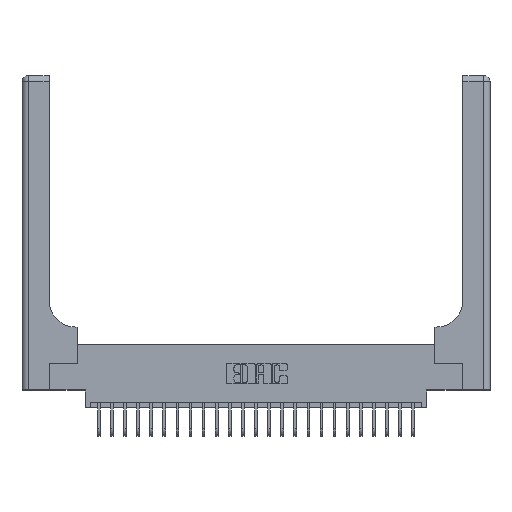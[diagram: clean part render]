
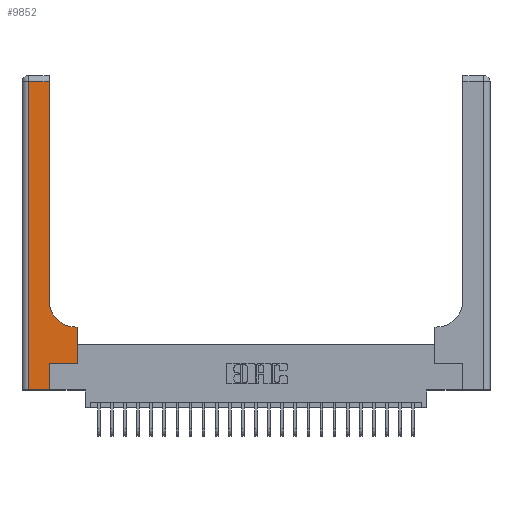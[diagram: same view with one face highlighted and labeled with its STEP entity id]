
A CAD part, top view. The second image highlights one B-rep face of the part: STEP entity #9852.
In plain terms, the highlighted planar face has unit normal (0, 0, 1).
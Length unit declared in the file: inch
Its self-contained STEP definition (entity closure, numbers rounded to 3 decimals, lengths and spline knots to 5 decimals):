
#57 = CARTESIAN_POINT ( 'NONE',  ( 0.06, 0., 0.37 ) ) ;
#827 = CARTESIAN_POINT ( 'NONE',  ( 0.26, 0.6, 0.37 ) ) ;
#976 = CARTESIAN_POINT ( 'NONE',  ( 0., 2.94, 0.37 ) ) ;
#1047 = DIRECTION ( 'NONE',  ( 0., 1., 0. ) ) ;
#1135 = DIRECTION ( 'NONE',  ( 0., 1., 0. ) ) ;
#1375 = LINE ( 'NONE', #8776, #22037 ) ;
#1558 = DIRECTION ( 'NONE',  ( 1., 0., 0. ) ) ;
#1727 = VERTEX_POINT ( 'NONE', #16387 ) ;
#2188 = VERTEX_POINT ( 'NONE', #4169 ) ;
#2196 = DIRECTION ( 'NONE',  ( 0., 1., 0. ) ) ;
#2370 = ORIENTED_EDGE ( 'NONE', *, *, #7358, .T. ) ;
#2479 = VERTEX_POINT ( 'NONE', #57 ) ;
#2896 = VECTOR ( 'NONE', #8259, 39.37008 ) ;
#3186 = ORIENTED_EDGE ( 'NONE', *, *, #9248, .T. ) ;
#3630 = ORIENTED_EDGE ( 'NONE', *, *, #19586, .T. ) ;
#3804 = CARTESIAN_POINT ( 'NONE',  ( 0.265, 0.25, 0.37 ) ) ;
#3867 = PLANE ( 'NONE',  #10212 ) ;
#4169 = CARTESIAN_POINT ( 'NONE',  ( 0.06, 2.94, 0.37 ) ) ;
#4468 = LINE ( 'NONE', #18923, #5776 ) ;
#4624 = VECTOR ( 'NONE', #9893, 39.37008 ) ;
#5185 = AXIS2_PLACEMENT_3D ( 'NONE', #12071, #22974, #1558 ) ;
#5554 = DIRECTION ( 'NONE',  ( -1., 0., 0. ) ) ;
#5571 = CARTESIAN_POINT ( 'NONE',  ( 0.265, 0., 0.37 ) ) ;
#5776 = VECTOR ( 'NONE', #2196, 39.37008 ) ;
#6435 = VERTEX_POINT ( 'NONE', #3804 ) ;
#6453 = CARTESIAN_POINT ( 'NONE',  ( 0.528, 0.25, 0.37 ) ) ;
#7325 = EDGE_CURVE ( 'NONE', #1727, #2188, #17358, .T. ) ;
#7358 = EDGE_CURVE ( 'NONE', #7975, #13155, #16233, .T. ) ;
#7469 = VERTEX_POINT ( 'NONE', #20322 ) ;
#7500 = VECTOR ( 'NONE', #1047, 39.37008 ) ;
#7531 = CARTESIAN_POINT ( 'NONE',  ( 0.26, 0.85, 0.37 ) ) ;
#7875 = LINE ( 'NONE', #827, #12632 ) ;
#7975 = VERTEX_POINT ( 'NONE', #10949 ) ;
#8026 = VECTOR ( 'NONE', #23571, 39.37008 ) ;
#8259 = DIRECTION ( 'NONE',  ( -1., 0., 0. ) ) ;
#8404 = ORIENTED_EDGE ( 'NONE', *, *, #15846, .T. ) ;
#8776 = CARTESIAN_POINT ( 'NONE',  ( 0.26, 3., 0.37 ) ) ;
#9248 = EDGE_CURVE ( 'NONE', #18885, #6435, #10131, .T. ) ;
#9634 = ORIENTED_EDGE ( 'NONE', *, *, #7325, .T. ) ;
#9682 = DIRECTION ( 'NONE',  ( -1., 0., 0. ) ) ;
#9770 = EDGE_CURVE ( 'NONE', #13155, #1727, #1375, .T. ) ;
#9852 = ADVANCED_FACE ( 'NONE', ( #21583 ), #3867, .F. ) ;
#9893 = DIRECTION ( 'NONE',  ( 1., 0., 0. ) ) ;
#10131 = LINE ( 'NONE', #21608, #7500 ) ;
#10212 = AXIS2_PLACEMENT_3D ( 'NONE', #11030, #12933, #5554 ) ;
#10528 = ORIENTED_EDGE ( 'NONE', *, *, #20988, .T. ) ;
#10949 = CARTESIAN_POINT ( 'NONE',  ( 0.51, 0.6, 0.37 ) ) ;
#11015 = CARTESIAN_POINT ( 'NONE',  ( 0.265, 0.25, 0.37 ) ) ;
#11030 = CARTESIAN_POINT ( 'NONE',  ( 0., 3., 0.37 ) ) ;
#11560 = LINE ( 'NONE', #18853, #4624 ) ;
#12071 = CARTESIAN_POINT ( 'NONE',  ( 0.51, 0.85, 0.37 ) ) ;
#12632 = VECTOR ( 'NONE', #9682, 39.37008 ) ;
#12933 = DIRECTION ( 'NONE',  ( 0., 0., -1. ) ) ;
#13155 = VERTEX_POINT ( 'NONE', #7531 ) ;
#13437 = VERTEX_POINT ( 'NONE', #6453 ) ;
#14504 = VECTOR ( 'NONE', #16527, 39.37008 ) ;
#15362 = ORIENTED_EDGE ( 'NONE', *, *, #21699, .T. ) ;
#15846 = EDGE_CURVE ( 'NONE', #7469, #7975, #7875, .T. ) ;
#16113 = ORIENTED_EDGE ( 'NONE', *, *, #23000, .T. ) ;
#16233 = CIRCLE ( 'NONE', #5185, 0.25 ) ;
#16387 = CARTESIAN_POINT ( 'NONE',  ( 0.26, 2.94, 0.37 ) ) ;
#16527 = DIRECTION ( 'NONE',  ( 1., 0., 0. ) ) ;
#16735 = EDGE_LOOP ( 'NONE', ( #21677, #9634, #3630, #10528, #3186, #15362, #16113, #8404, #2370 ) ) ;
#17358 = LINE ( 'NONE', #976, #2896 ) ;
#17942 = LINE ( 'NONE', #23454, #8026 ) ;
#18853 = CARTESIAN_POINT ( 'NONE',  ( 0., 0., 0.37 ) ) ;
#18885 = VERTEX_POINT ( 'NONE', #5571 ) ;
#18923 = CARTESIAN_POINT ( 'NONE',  ( 0.528, 0.25, 0.37 ) ) ;
#19586 = EDGE_CURVE ( 'NONE', #2188, #2479, #17942, .T. ) ;
#20322 = CARTESIAN_POINT ( 'NONE',  ( 0.528, 0.6, 0.37 ) ) ;
#20988 = EDGE_CURVE ( 'NONE', #2479, #18885, #11560, .T. ) ;
#21583 = FACE_OUTER_BOUND ( 'NONE', #16735, .T. ) ;
#21608 = CARTESIAN_POINT ( 'NONE',  ( 0.265, 0., 0.37 ) ) ;
#21677 = ORIENTED_EDGE ( 'NONE', *, *, #9770, .T. ) ;
#21685 = LINE ( 'NONE', #11015, #14504 ) ;
#21699 = EDGE_CURVE ( 'NONE', #6435, #13437, #21685, .T. ) ;
#22037 = VECTOR ( 'NONE', #1135, 39.37008 ) ;
#22974 = DIRECTION ( 'NONE',  ( 0., 0., -1. ) ) ;
#23000 = EDGE_CURVE ( 'NONE', #13437, #7469, #4468, .T. ) ;
#23454 = CARTESIAN_POINT ( 'NONE',  ( 0.06, 3., 0.37 ) ) ;
#23571 = DIRECTION ( 'NONE',  ( 0., -1., 0. ) ) ;
